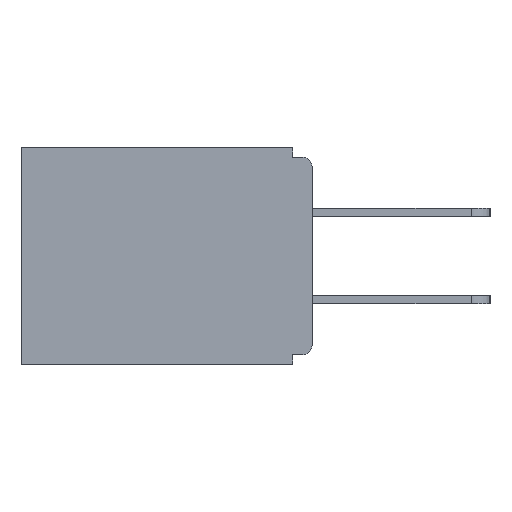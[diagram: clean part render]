
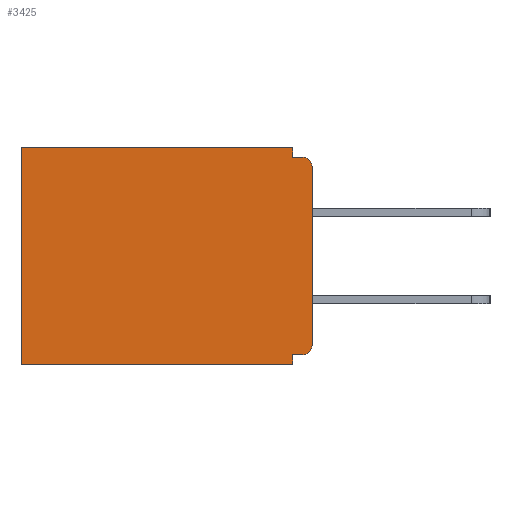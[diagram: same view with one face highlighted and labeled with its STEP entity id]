
A CAD part, left-side view. The second image highlights one B-rep face of the part: STEP entity #3425.
In plain terms, the highlighted planar face has unit normal (-1, 0, 0).
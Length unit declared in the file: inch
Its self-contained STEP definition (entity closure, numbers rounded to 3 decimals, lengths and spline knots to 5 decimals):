
#60 = CARTESIAN_POINT ( 'NONE',  ( 0.298, 0.031, -0.015 ) ) ;
#334 = VERTEX_POINT ( 'NONE', #21173 ) ;
#377 = CARTESIAN_POINT ( 'NONE',  ( 0.298, 0., 0. ) ) ;
#1606 = CARTESIAN_POINT ( 'NONE',  ( 0.298, 0.031, 0. ) ) ;
#1838 = CARTESIAN_POINT ( 'NONE',  ( 0.298, 0., -0.015 ) ) ;
#1937 = ORIENTED_EDGE ( 'NONE', *, *, #2247, .F. ) ;
#2247 = EDGE_CURVE ( 'NONE', #17313, #10667, #20907, .T. ) ;
#2853 = LINE ( 'NONE', #13103, #8628 ) ;
#3055 = VECTOR ( 'NONE', #27398, 39.37008 ) ;
#3425 = ADVANCED_FACE ( 'NONE', ( #8910 ), #27975, .F. ) ;
#3744 = CARTESIAN_POINT ( 'NONE',  ( 0.298, 0.46, 0. ) ) ;
#4092 = VERTEX_POINT ( 'NONE', #15533 ) ;
#4311 = VERTEX_POINT ( 'NONE', #26295 ) ;
#4371 = EDGE_CURVE ( 'NONE', #334, #28335, #25839, .T. ) ;
#5600 = CARTESIAN_POINT ( 'NONE',  ( 0.298, 0., -0.313 ) ) ;
#5637 = DIRECTION ( 'NONE',  ( 0., 1., 0. ) ) ;
#5694 = ORIENTED_EDGE ( 'NONE', *, *, #18045, .F. ) ;
#5821 = VECTOR ( 'NONE', #22578, 39.37008 ) ;
#6232 = ORIENTED_EDGE ( 'NONE', *, *, #21705, .F. ) ;
#6292 = ORIENTED_EDGE ( 'NONE', *, *, #29637, .T. ) ;
#8628 = VECTOR ( 'NONE', #17445, 39.37008 ) ;
#8650 = DIRECTION ( 'NONE',  ( -1., 0., 0. ) ) ;
#8760 = EDGE_CURVE ( 'NONE', #334, #4092, #29580, .T. ) ;
#8854 = ORIENTED_EDGE ( 'NONE', *, *, #15016, .T. ) ;
#8910 = FACE_OUTER_BOUND ( 'NONE', #11202, .T. ) ;
#10426 = EDGE_CURVE ( 'NONE', #4311, #22191, #25876, .T. ) ;
#10667 = VERTEX_POINT ( 'NONE', #15192 ) ;
#10900 = ORIENTED_EDGE ( 'NONE', *, *, #4371, .T. ) ;
#11176 = LINE ( 'NONE', #22153, #28854 ) ;
#11202 = EDGE_LOOP ( 'NONE', ( #23355, #12355, #5694, #6292, #8854, #1937, #6232, #12931, #10900, #17564 ) ) ;
#12031 = LINE ( 'NONE', #3744, #14150 ) ;
#12156 = DIRECTION ( 'NONE',  ( 0., 0., -1. ) ) ;
#12327 = DIRECTION ( 'NONE',  ( 0., 0., -1. ) ) ;
#12355 = ORIENTED_EDGE ( 'NONE', *, *, #16121, .F. ) ;
#12797 = CARTESIAN_POINT ( 'NONE',  ( 0.298, 0., -0.328 ) ) ;
#12931 = ORIENTED_EDGE ( 'NONE', *, *, #8760, .F. ) ;
#13103 = CARTESIAN_POINT ( 'NONE',  ( 0.298, 0.031, -0.343 ) ) ;
#13667 = AXIS2_PLACEMENT_3D ( 'NONE', #19040, #26007, #12156 ) ;
#14150 = VECTOR ( 'NONE', #24426, 39.37008 ) ;
#15016 = EDGE_CURVE ( 'NONE', #18963, #10667, #12031, .T. ) ;
#15192 = CARTESIAN_POINT ( 'NONE',  ( 0.298, 0.46, -0.343 ) ) ;
#15533 = CARTESIAN_POINT ( 'NONE',  ( 0.298, 0.031, -0.328 ) ) ;
#15589 = DIRECTION ( 'NONE',  ( 0., 0., -1. ) ) ;
#16083 = CARTESIAN_POINT ( 'NONE',  ( 0.298, 0., 0. ) ) ;
#16121 = EDGE_CURVE ( 'NONE', #24047, #22191, #20642, .T. ) ;
#16484 = DIRECTION ( 'NONE',  ( 1., 0., 0. ) ) ;
#16539 = VECTOR ( 'NONE', #21001, 39.37008 ) ;
#17313 = VERTEX_POINT ( 'NONE', #18290 ) ;
#17445 = DIRECTION ( 'NONE',  ( 0., 0., -1. ) ) ;
#17564 = ORIENTED_EDGE ( 'NONE', *, *, #29457, .F. ) ;
#18045 = EDGE_CURVE ( 'NONE', #22693, #24047, #2853, .T. ) ;
#18290 = CARTESIAN_POINT ( 'NONE',  ( 0.298, 0.031, -0.343 ) ) ;
#18963 = VERTEX_POINT ( 'NONE', #22780 ) ;
#19005 = CARTESIAN_POINT ( 'NONE',  ( 0.298, 0., 0. ) ) ;
#19040 = CARTESIAN_POINT ( 'NONE',  ( 0.298, 0.015, -0.03 ) ) ;
#19102 = AXIS2_PLACEMENT_3D ( 'NONE', #24581, #8650, #15589 ) ;
#19963 = CARTESIAN_POINT ( 'NONE',  ( 0.298, 0.015, -0.015 ) ) ;
#20642 = LINE ( 'NONE', #1838, #5821 ) ;
#20761 = LINE ( 'NONE', #16083, #3055 ) ;
#20907 = LINE ( 'NONE', #23409, #16539 ) ;
#21001 = DIRECTION ( 'NONE',  ( 0., 1., 0. ) ) ;
#21125 = DIRECTION ( 'NONE',  ( 0., 1., 0. ) ) ;
#21173 = CARTESIAN_POINT ( 'NONE',  ( 0.298, 0.015, -0.328 ) ) ;
#21453 = VECTOR ( 'NONE', #21125, 39.37008 ) ;
#21705 = EDGE_CURVE ( 'NONE', #4092, #17313, #11176, .T. ) ;
#22153 = CARTESIAN_POINT ( 'NONE',  ( 0.298, 0.031, -0.343 ) ) ;
#22191 = VERTEX_POINT ( 'NONE', #19963 ) ;
#22578 = DIRECTION ( 'NONE',  ( 0., -1., 0. ) ) ;
#22693 = VERTEX_POINT ( 'NONE', #1606 ) ;
#22780 = CARTESIAN_POINT ( 'NONE',  ( 0.298, 0.46, 0. ) ) ;
#23355 = ORIENTED_EDGE ( 'NONE', *, *, #10426, .T. ) ;
#23409 = CARTESIAN_POINT ( 'NONE',  ( 0.298, 0., -0.343 ) ) ;
#24047 = VERTEX_POINT ( 'NONE', #60 ) ;
#24426 = DIRECTION ( 'NONE',  ( 0., 0., -1. ) ) ;
#24491 = DIRECTION ( 'NONE',  ( 0., 0., -1. ) ) ;
#24581 = CARTESIAN_POINT ( 'NONE',  ( 0.298, 0.015, -0.313 ) ) ;
#25839 = CIRCLE ( 'NONE', #19102, 0.015 ) ;
#25876 = CIRCLE ( 'NONE', #13667, 0.015 ) ;
#26007 = DIRECTION ( 'NONE',  ( -1., 0., 0. ) ) ;
#26044 = AXIS2_PLACEMENT_3D ( 'NONE', #377, #16484, #12327 ) ;
#26295 = CARTESIAN_POINT ( 'NONE',  ( 0.298, 0., -0.03 ) ) ;
#26337 = VECTOR ( 'NONE', #5637, 39.37008 ) ;
#27398 = DIRECTION ( 'NONE',  ( 0., 0., -1. ) ) ;
#27975 = PLANE ( 'NONE',  #26044 ) ;
#28294 = LINE ( 'NONE', #19005, #21453 ) ;
#28335 = VERTEX_POINT ( 'NONE', #5600 ) ;
#28854 = VECTOR ( 'NONE', #24491, 39.37008 ) ;
#29457 = EDGE_CURVE ( 'NONE', #4311, #28335, #20761, .T. ) ;
#29580 = LINE ( 'NONE', #12797, #26337 ) ;
#29637 = EDGE_CURVE ( 'NONE', #22693, #18963, #28294, .T. ) ;
